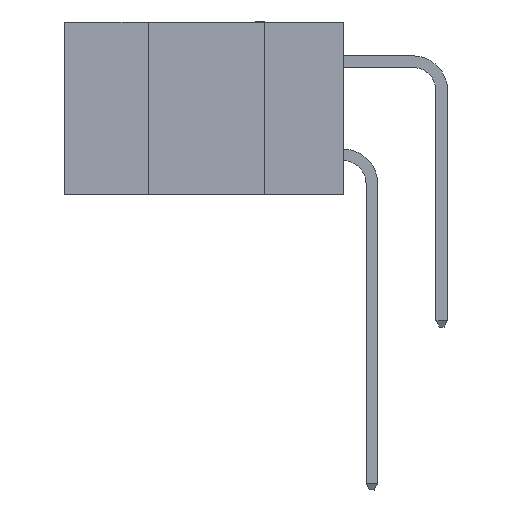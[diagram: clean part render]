
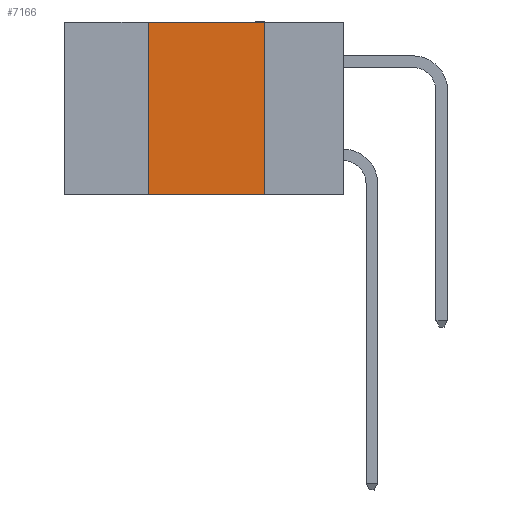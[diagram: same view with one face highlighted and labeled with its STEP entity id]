
A CAD part, left-side view. The second image highlights one B-rep face of the part: STEP entity #7166.
In plain terms, the highlighted planar face has unit normal (-1, 0, 0).
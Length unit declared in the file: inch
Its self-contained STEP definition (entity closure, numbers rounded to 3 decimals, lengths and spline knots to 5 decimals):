
#381 = VECTOR ( 'NONE', #4650, 39.37008 ) ;
#1091 = CARTESIAN_POINT ( 'NONE',  ( 0., 0.6, -0.37 ) ) ;
#1093 = FACE_OUTER_BOUND ( 'NONE', #19325, .T. ) ;
#2090 = CARTESIAN_POINT ( 'NONE',  ( 0., 0.6, 0. ) ) ;
#2210 = EDGE_CURVE ( 'NONE', #16231, #8190, #4410, .T. ) ;
#2799 = CARTESIAN_POINT ( 'NONE',  ( 0., 0.6, 0. ) ) ;
#3139 = DIRECTION ( 'NONE',  ( 1., 0., 0. ) ) ;
#3804 = CARTESIAN_POINT ( 'NONE',  ( 0., 0.17, 0. ) ) ;
#4258 = DIRECTION ( 'NONE',  ( 0., -1., 0. ) ) ;
#4410 = LINE ( 'NONE', #1091, #381 ) ;
#4650 = DIRECTION ( 'NONE',  ( 0., -1., 0. ) ) ;
#5174 = CARTESIAN_POINT ( 'NONE',  ( 0., 0.42, 0. ) ) ;
#5442 = CARTESIAN_POINT ( 'NONE',  ( 0., 0.17, 0. ) ) ;
#5676 = EDGE_CURVE ( 'NONE', #21622, #14602, #21137, .T. ) ;
#6398 = DIRECTION ( 'NONE',  ( 0., 0., -1. ) ) ;
#6728 = AXIS2_PLACEMENT_3D ( 'NONE', #2799, #3139, #6398 ) ;
#7166 = ADVANCED_FACE ( 'NONE', ( #1093 ), #22692, .F. ) ;
#8190 = VERTEX_POINT ( 'NONE', #10321 ) ;
#9345 = VECTOR ( 'NONE', #13545, 39.37008 ) ;
#9672 = LINE ( 'NONE', #3804, #9345 ) ;
#10321 = CARTESIAN_POINT ( 'NONE',  ( 0., 0.17, -0.37 ) ) ;
#10808 = LINE ( 'NONE', #12378, #17532 ) ;
#12378 = CARTESIAN_POINT ( 'NONE',  ( 0., 0.42, 0. ) ) ;
#13276 = ORIENTED_EDGE ( 'NONE', *, *, #21067, .F. ) ;
#13545 = DIRECTION ( 'NONE',  ( 0., 0., -1. ) ) ;
#14602 = VERTEX_POINT ( 'NONE', #5442 ) ;
#15615 = CARTESIAN_POINT ( 'NONE',  ( 0., 0.42, -0.37 ) ) ;
#16231 = VERTEX_POINT ( 'NONE', #15615 ) ;
#16921 = DIRECTION ( 'NONE',  ( 0., 0., 1. ) ) ;
#16924 = ORIENTED_EDGE ( 'NONE', *, *, #2210, .T. ) ;
#17532 = VECTOR ( 'NONE', #16921, 39.37008 ) ;
#19325 = EDGE_LOOP ( 'NONE', ( #24116, #23635, #13276, #16924 ) ) ;
#21067 = EDGE_CURVE ( 'NONE', #16231, #21622, #10808, .T. ) ;
#21137 = LINE ( 'NONE', #2090, #21433 ) ;
#21433 = VECTOR ( 'NONE', #4258, 39.37008 ) ;
#21622 = VERTEX_POINT ( 'NONE', #5174 ) ;
#22692 = PLANE ( 'NONE',  #6728 ) ;
#23635 = ORIENTED_EDGE ( 'NONE', *, *, #5676, .F. ) ;
#24116 = ORIENTED_EDGE ( 'NONE', *, *, #24710, .F. ) ;
#24710 = EDGE_CURVE ( 'NONE', #14602, #8190, #9672, .T. ) ;
